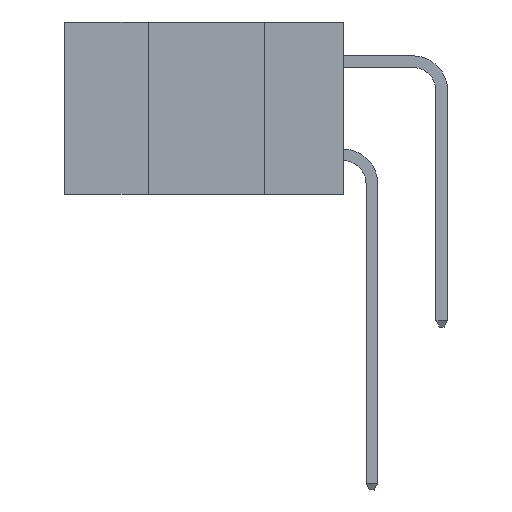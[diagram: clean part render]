
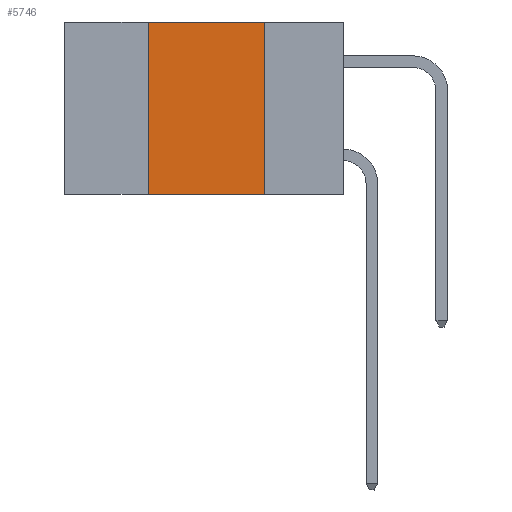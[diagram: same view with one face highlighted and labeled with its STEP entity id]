
A CAD part, left-side view. The second image highlights one B-rep face of the part: STEP entity #5746.
In plain terms, the highlighted planar face has unit normal (-1, 0, 0).
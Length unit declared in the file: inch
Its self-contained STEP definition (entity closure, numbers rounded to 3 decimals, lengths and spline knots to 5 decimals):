
#69 = VECTOR ( 'NONE', #26094, 39.37008 ) ;
#334 = CARTESIAN_POINT ( 'NONE',  ( 0., 0.42, 0. ) ) ;
#1883 = CARTESIAN_POINT ( 'NONE',  ( 0., 0.42, -0.37 ) ) ;
#4410 = LINE ( 'NONE', #19315, #24194 ) ;
#5706 = DIRECTION ( 'NONE',  ( 0., 0., -1. ) ) ;
#5746 = ADVANCED_FACE ( 'NONE', ( #20425 ), #18268, .F. ) ;
#5775 = LINE ( 'NONE', #8519, #22969 ) ;
#6519 = EDGE_LOOP ( 'NONE', ( #13807, #16466, #16992, #9862 ) ) ;
#8519 = CARTESIAN_POINT ( 'NONE',  ( 0., 0.6, -0.37 ) ) ;
#9862 = ORIENTED_EDGE ( 'NONE', *, *, #19288, .T. ) ;
#10081 = CARTESIAN_POINT ( 'NONE',  ( 0., 0.6, 0. ) ) ;
#10668 = CARTESIAN_POINT ( 'NONE',  ( 0., 0.17, -0.37 ) ) ;
#10921 = LINE ( 'NONE', #10081, #19788 ) ;
#11101 = VERTEX_POINT ( 'NONE', #1883 ) ;
#12108 = CARTESIAN_POINT ( 'NONE',  ( 0., 0.6, 0. ) ) ;
#12421 = VERTEX_POINT ( 'NONE', #26919 ) ;
#13363 = EDGE_CURVE ( 'NONE', #12421, #25311, #4410, .T. ) ;
#13807 = ORIENTED_EDGE ( 'NONE', *, *, #13363, .F. ) ;
#15276 = DIRECTION ( 'NONE',  ( 0., 0., -1. ) ) ;
#16466 = ORIENTED_EDGE ( 'NONE', *, *, #26150, .F. ) ;
#16992 = ORIENTED_EDGE ( 'NONE', *, *, #21310, .F. ) ;
#17251 = DIRECTION ( 'NONE',  ( 0., -1., 0. ) ) ;
#18268 = PLANE ( 'NONE',  #18654 ) ;
#18540 = DIRECTION ( 'NONE',  ( 0., -1., 0. ) ) ;
#18654 = AXIS2_PLACEMENT_3D ( 'NONE', #12108, #22667, #5706 ) ;
#19288 = EDGE_CURVE ( 'NONE', #11101, #25311, #5775, .T. ) ;
#19315 = CARTESIAN_POINT ( 'NONE',  ( 0., 0.17, 0. ) ) ;
#19788 = VECTOR ( 'NONE', #18540, 39.37008 ) ;
#20425 = FACE_OUTER_BOUND ( 'NONE', #6519, .T. ) ;
#21200 = LINE ( 'NONE', #22118, #69 ) ;
#21310 = EDGE_CURVE ( 'NONE', #11101, #23468, #21200, .T. ) ;
#22118 = CARTESIAN_POINT ( 'NONE',  ( 0., 0.42, 0. ) ) ;
#22667 = DIRECTION ( 'NONE',  ( 1., 0., 0. ) ) ;
#22969 = VECTOR ( 'NONE', #17251, 39.37008 ) ;
#23468 = VERTEX_POINT ( 'NONE', #334 ) ;
#24194 = VECTOR ( 'NONE', #15276, 39.37008 ) ;
#25311 = VERTEX_POINT ( 'NONE', #10668 ) ;
#26094 = DIRECTION ( 'NONE',  ( 0., 0., 1. ) ) ;
#26150 = EDGE_CURVE ( 'NONE', #23468, #12421, #10921, .T. ) ;
#26919 = CARTESIAN_POINT ( 'NONE',  ( 0., 0.17, 0. ) ) ;
